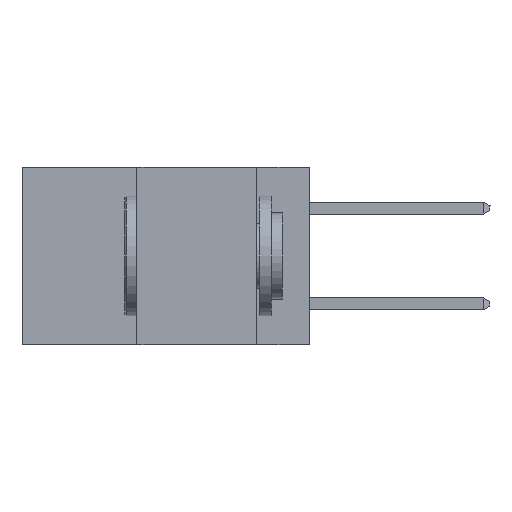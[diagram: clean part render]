
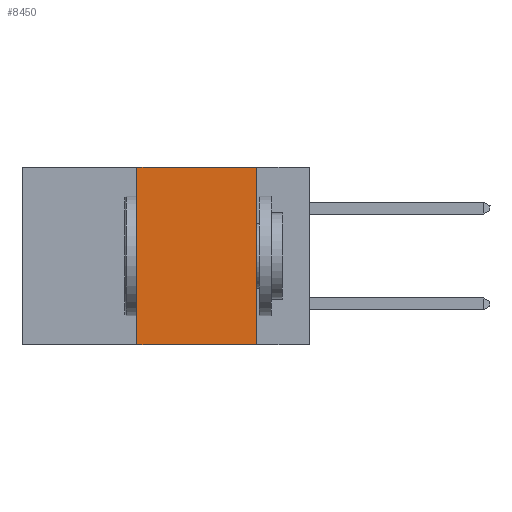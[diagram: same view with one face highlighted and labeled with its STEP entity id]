
A CAD part, left-side view. The second image highlights one B-rep face of the part: STEP entity #8450.
In plain terms, the highlighted planar face has unit normal (-1, 0, 0).
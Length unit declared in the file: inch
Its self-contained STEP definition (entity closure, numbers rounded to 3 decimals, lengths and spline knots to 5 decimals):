
#148 = VECTOR ( 'NONE', #11407, 39.37008 ) ;
#205 = ORIENTED_EDGE ( 'NONE', *, *, #12262, .T. ) ;
#351 = EDGE_LOOP ( 'NONE', ( #3729, #2301, #12454, #205 ) ) ;
#864 = LINE ( 'NONE', #1817, #13610 ) ;
#1634 = LINE ( 'NONE', #3399, #148 ) ;
#1817 = CARTESIAN_POINT ( 'NONE',  ( 0., 0.36, 0. ) ) ;
#2109 = VERTEX_POINT ( 'NONE', #7048 ) ;
#2301 = ORIENTED_EDGE ( 'NONE', *, *, #7450, .F. ) ;
#3346 = VECTOR ( 'NONE', #14451, 39.37008 ) ;
#3399 = CARTESIAN_POINT ( 'NONE',  ( 0., 0.6, 0. ) ) ;
#3729 = ORIENTED_EDGE ( 'NONE', *, *, #14353, .F. ) ;
#3894 = CARTESIAN_POINT ( 'NONE',  ( 0., 0.6, 0. ) ) ;
#6116 = DIRECTION ( 'NONE',  ( 0., 0., -1. ) ) ;
#6166 = DIRECTION ( 'NONE',  ( 1., 0., 0. ) ) ;
#6388 = CARTESIAN_POINT ( 'NONE',  ( 0., 0.6, -0.37 ) ) ;
#6644 = CARTESIAN_POINT ( 'NONE',  ( 0., 0.11, 0. ) ) ;
#7048 = CARTESIAN_POINT ( 'NONE',  ( 0., 0.11, -0.37 ) ) ;
#7450 = EDGE_CURVE ( 'NONE', #11725, #9037, #1634, .T. ) ;
#7835 = LINE ( 'NONE', #6388, #3346 ) ;
#8450 = ADVANCED_FACE ( 'NONE', ( #9747 ), #11879, .F. ) ;
#9024 = LINE ( 'NONE', #6644, #9390 ) ;
#9037 = VERTEX_POINT ( 'NONE', #12659 ) ;
#9390 = VECTOR ( 'NONE', #13490, 39.37008 ) ;
#9747 = FACE_OUTER_BOUND ( 'NONE', #351, .T. ) ;
#10475 = VERTEX_POINT ( 'NONE', #11312 ) ;
#10843 = AXIS2_PLACEMENT_3D ( 'NONE', #3894, #6166, #6116 ) ;
#11312 = CARTESIAN_POINT ( 'NONE',  ( 0., 0.36, -0.37 ) ) ;
#11407 = DIRECTION ( 'NONE',  ( 0., -1., 0. ) ) ;
#11451 = EDGE_CURVE ( 'NONE', #10475, #11725, #864, .T. ) ;
#11725 = VERTEX_POINT ( 'NONE', #13869 ) ;
#11879 = PLANE ( 'NONE',  #10843 ) ;
#12222 = DIRECTION ( 'NONE',  ( 0., 0., 1. ) ) ;
#12262 = EDGE_CURVE ( 'NONE', #10475, #2109, #7835, .T. ) ;
#12454 = ORIENTED_EDGE ( 'NONE', *, *, #11451, .F. ) ;
#12659 = CARTESIAN_POINT ( 'NONE',  ( 0., 0.11, 0. ) ) ;
#13490 = DIRECTION ( 'NONE',  ( 0., 0., -1. ) ) ;
#13610 = VECTOR ( 'NONE', #12222, 39.37008 ) ;
#13869 = CARTESIAN_POINT ( 'NONE',  ( 0., 0.36, 0. ) ) ;
#14353 = EDGE_CURVE ( 'NONE', #9037, #2109, #9024, .T. ) ;
#14451 = DIRECTION ( 'NONE',  ( 0., -1., 0. ) ) ;
